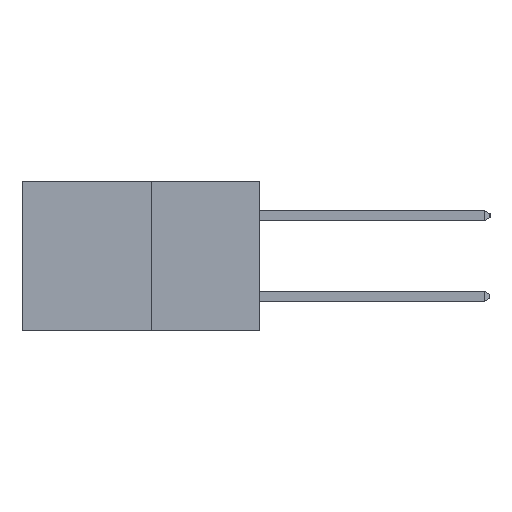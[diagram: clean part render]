
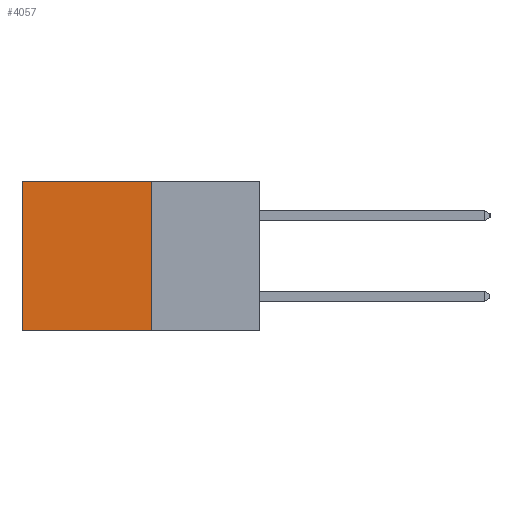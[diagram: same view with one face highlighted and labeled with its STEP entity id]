
A CAD part, left-side view. The second image highlights one B-rep face of the part: STEP entity #4057.
In plain terms, the highlighted planar face has unit normal (-1, 0, 0).
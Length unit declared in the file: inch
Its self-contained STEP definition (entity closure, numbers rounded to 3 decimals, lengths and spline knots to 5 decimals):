
#24 = VECTOR ( 'NONE', #1628, 39.37008 ) ;
#259 = DIRECTION ( 'NONE',  ( 0., 0., -1. ) ) ;
#284 = PLANE ( 'NONE',  #3600 ) ;
#306 = DIRECTION ( 'NONE',  ( 0., 1., 0. ) ) ;
#315 = VERTEX_POINT ( 'NONE', #7071 ) ;
#694 = ORIENTED_EDGE ( 'NONE', *, *, #1541, .F. ) ;
#1158 = LINE ( 'NONE', #5371, #6647 ) ;
#1541 = EDGE_CURVE ( 'NONE', #315, #4161, #1158, .T. ) ;
#1628 = DIRECTION ( 'NONE',  ( 0., 1., 0. ) ) ;
#1633 = CARTESIAN_POINT ( 'NONE',  ( 0.277, 0.27, -0.37 ) ) ;
#1711 = EDGE_CURVE ( 'NONE', #315, #1863, #5879, .T. ) ;
#1863 = VERTEX_POINT ( 'NONE', #5634 ) ;
#2215 = CARTESIAN_POINT ( 'NONE',  ( 0.277, 0.59, -0.37 ) ) ;
#2240 = DIRECTION ( 'NONE',  ( 0., 0., -1. ) ) ;
#2614 = CARTESIAN_POINT ( 'NONE',  ( 0.277, 0.27, 0. ) ) ;
#2812 = EDGE_LOOP ( 'NONE', ( #6527, #4329, #694, #6431 ) ) ;
#3600 = AXIS2_PLACEMENT_3D ( 'NONE', #6844, #6761, #259 ) ;
#3618 = LINE ( 'NONE', #1633, #24 ) ;
#3653 = DIRECTION ( 'NONE',  ( 0., 0., -1. ) ) ;
#4057 = ADVANCED_FACE ( 'NONE', ( #8793 ), #284, .F. ) ;
#4161 = VERTEX_POINT ( 'NONE', #6853 ) ;
#4329 = ORIENTED_EDGE ( 'NONE', *, *, #6819, .F. ) ;
#4470 = VECTOR ( 'NONE', #2240, 39.37008 ) ;
#5371 = CARTESIAN_POINT ( 'NONE',  ( 0.277, 0.27, -0.37 ) ) ;
#5634 = CARTESIAN_POINT ( 'NONE',  ( 0.277, 0.59, 0. ) ) ;
#5879 = LINE ( 'NONE', #2614, #7713 ) ;
#6232 = VERTEX_POINT ( 'NONE', #6609 ) ;
#6431 = ORIENTED_EDGE ( 'NONE', *, *, #1711, .T. ) ;
#6527 = ORIENTED_EDGE ( 'NONE', *, *, #6769, .T. ) ;
#6609 = CARTESIAN_POINT ( 'NONE',  ( 0.277, 0.59, -0.37 ) ) ;
#6647 = VECTOR ( 'NONE', #3653, 39.37008 ) ;
#6761 = DIRECTION ( 'NONE',  ( 1., 0., 0. ) ) ;
#6769 = EDGE_CURVE ( 'NONE', #1863, #6232, #8119, .T. ) ;
#6819 = EDGE_CURVE ( 'NONE', #4161, #6232, #3618, .T. ) ;
#6844 = CARTESIAN_POINT ( 'NONE',  ( 0.277, 0.27, -0.37 ) ) ;
#6853 = CARTESIAN_POINT ( 'NONE',  ( 0.277, 0.27, -0.37 ) ) ;
#7071 = CARTESIAN_POINT ( 'NONE',  ( 0.277, 0.27, 0. ) ) ;
#7713 = VECTOR ( 'NONE', #306, 39.37008 ) ;
#8119 = LINE ( 'NONE', #2215, #4470 ) ;
#8793 = FACE_OUTER_BOUND ( 'NONE', #2812, .T. ) ;
